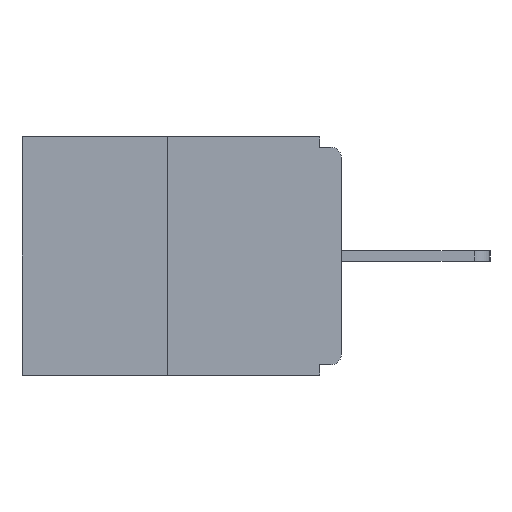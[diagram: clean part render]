
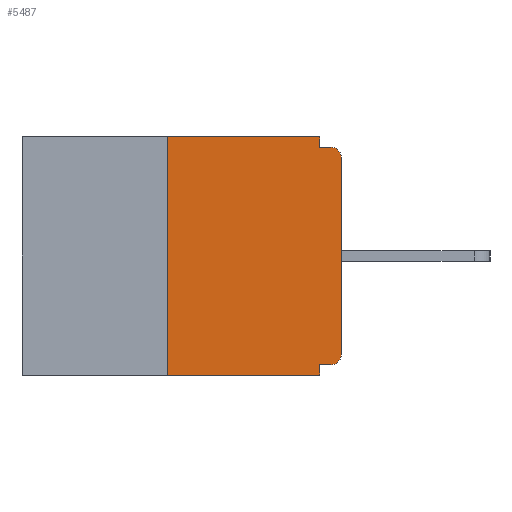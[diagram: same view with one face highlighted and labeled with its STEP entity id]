
A CAD part, left-side view. The second image highlights one B-rep face of the part: STEP entity #5487.
In plain terms, the highlighted planar face has unit normal (-1, 0, 0).
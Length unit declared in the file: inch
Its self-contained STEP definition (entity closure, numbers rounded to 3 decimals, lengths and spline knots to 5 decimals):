
#47 = CARTESIAN_POINT ( 'NONE',  ( 0., 0.015, -0.328 ) ) ;
#153 = CARTESIAN_POINT ( 'NONE',  ( 0., 0., -0.328 ) ) ;
#183 = CARTESIAN_POINT ( 'NONE',  ( 0., 0.46, 0. ) ) ;
#528 = EDGE_CURVE ( 'NONE', #22806, #22956, #4573, .T. ) ;
#566 = CARTESIAN_POINT ( 'NONE',  ( 0., 0., -0.015 ) ) ;
#875 = CARTESIAN_POINT ( 'NONE',  ( 0., 0.031, -0.015 ) ) ;
#1063 = ORIENTED_EDGE ( 'NONE', *, *, #13014, .T. ) ;
#1598 = CIRCLE ( 'NONE', #15785, 0.015 ) ;
#1713 = LINE ( 'NONE', #566, #11301 ) ;
#2596 = ORIENTED_EDGE ( 'NONE', *, *, #18009, .F. ) ;
#2713 = VERTEX_POINT ( 'NONE', #8133 ) ;
#3279 = CARTESIAN_POINT ( 'NONE',  ( 0., 0.031, 0. ) ) ;
#3732 = PLANE ( 'NONE',  #17270 ) ;
#3936 = EDGE_CURVE ( 'NONE', #22615, #22133, #1598, .T. ) ;
#4573 = LINE ( 'NONE', #6725, #20364 ) ;
#4739 = CARTESIAN_POINT ( 'NONE',  ( 0., 0., -0.03 ) ) ;
#4906 = DIRECTION ( 'NONE',  ( 0., 0., -1. ) ) ;
#4944 = DIRECTION ( 'NONE',  ( 0., -1., 0. ) ) ;
#5303 = CARTESIAN_POINT ( 'NONE',  ( 0., 0.015, -0.03 ) ) ;
#5355 = DIRECTION ( 'NONE',  ( -1., 0., 0. ) ) ;
#5487 = ADVANCED_FACE ( 'NONE', ( #7927 ), #3732, .F. ) ;
#5621 = LINE ( 'NONE', #18675, #11233 ) ;
#5684 = DIRECTION ( 'NONE',  ( 0., 0., -1. ) ) ;
#5750 = VERTEX_POINT ( 'NONE', #8669 ) ;
#5790 = VECTOR ( 'NONE', #16634, 39.37008 ) ;
#6542 = EDGE_CURVE ( 'NONE', #11334, #2713, #22577, .T. ) ;
#6725 = CARTESIAN_POINT ( 'NONE',  ( 0., 0.46, 0. ) ) ;
#6993 = CARTESIAN_POINT ( 'NONE',  ( 0., 0.46, -0.343 ) ) ;
#7235 = CARTESIAN_POINT ( 'NONE',  ( 0., 0.031, -0.328 ) ) ;
#7927 = FACE_OUTER_BOUND ( 'NONE', #17029, .T. ) ;
#7964 = EDGE_CURVE ( 'NONE', #22956, #19460, #20913, .T. ) ;
#8133 = CARTESIAN_POINT ( 'NONE',  ( 0., 0., -0.313 ) ) ;
#8654 = ORIENTED_EDGE ( 'NONE', *, *, #14300, .F. ) ;
#8669 = CARTESIAN_POINT ( 'NONE',  ( 0., 0.25, -0.343 ) ) ;
#9293 = LINE ( 'NONE', #153, #14340 ) ;
#10067 = VERTEX_POINT ( 'NONE', #15143 ) ;
#10316 = EDGE_CURVE ( 'NONE', #19460, #22133, #1713, .T. ) ;
#10965 = DIRECTION ( 'NONE',  ( 0., 0., -1. ) ) ;
#11146 = DIRECTION ( 'NONE',  ( 0., 0., 1. ) ) ;
#11233 = VECTOR ( 'NONE', #10965, 39.37008 ) ;
#11301 = VECTOR ( 'NONE', #14036, 39.37008 ) ;
#11334 = VERTEX_POINT ( 'NONE', #47 ) ;
#11351 = LINE ( 'NONE', #18862, #15812 ) ;
#11620 = ORIENTED_EDGE ( 'NONE', *, *, #10316, .F. ) ;
#11762 = EDGE_CURVE ( 'NONE', #18488, #10067, #5621, .T. ) ;
#13014 = EDGE_CURVE ( 'NONE', #5750, #10067, #18652, .T. ) ;
#13365 = ORIENTED_EDGE ( 'NONE', *, *, #6542, .T. ) ;
#14036 = DIRECTION ( 'NONE',  ( 0., -1., 0. ) ) ;
#14300 = EDGE_CURVE ( 'NONE', #5750, #22806, #21024, .T. ) ;
#14340 = VECTOR ( 'NONE', #19371, 39.37008 ) ;
#15002 = DIRECTION ( 'NONE',  ( 0., 0., 1. ) ) ;
#15143 = CARTESIAN_POINT ( 'NONE',  ( 0., 0.031, -0.343 ) ) ;
#15548 = DIRECTION ( 'NONE',  ( 0., 0., -1. ) ) ;
#15574 = DIRECTION ( 'NONE',  ( -1., 0., 0. ) ) ;
#15600 = CARTESIAN_POINT ( 'NONE',  ( 0., 0.015, -0.313 ) ) ;
#15785 = AXIS2_PLACEMENT_3D ( 'NONE', #5303, #5355, #5684 ) ;
#15812 = VECTOR ( 'NONE', #15002, 39.37008 ) ;
#16568 = VECTOR ( 'NONE', #11146, 39.37008 ) ;
#16634 = DIRECTION ( 'NONE',  ( 0., 0., -1. ) ) ;
#17029 = EDGE_LOOP ( 'NONE', ( #18161, #8654, #1063, #17575, #2596, #13365, #24479, #18791, #11620, #20601 ) ) ;
#17217 = CARTESIAN_POINT ( 'NONE',  ( 0., 0.031, 0. ) ) ;
#17270 = AXIS2_PLACEMENT_3D ( 'NONE', #183, #23606, #4906 ) ;
#17575 = ORIENTED_EDGE ( 'NONE', *, *, #11762, .F. ) ;
#18009 = EDGE_CURVE ( 'NONE', #11334, #18488, #9293, .T. ) ;
#18161 = ORIENTED_EDGE ( 'NONE', *, *, #528, .F. ) ;
#18488 = VERTEX_POINT ( 'NONE', #7235 ) ;
#18652 = LINE ( 'NONE', #6993, #22352 ) ;
#18654 = CARTESIAN_POINT ( 'NONE',  ( 0., 0.25, 0. ) ) ;
#18675 = CARTESIAN_POINT ( 'NONE',  ( 0., 0.031, -0.343 ) ) ;
#18791 = ORIENTED_EDGE ( 'NONE', *, *, #3936, .T. ) ;
#18862 = CARTESIAN_POINT ( 'NONE',  ( 0., 0., 0. ) ) ;
#19371 = DIRECTION ( 'NONE',  ( 0., 1., 0. ) ) ;
#19460 = VERTEX_POINT ( 'NONE', #875 ) ;
#20364 = VECTOR ( 'NONE', #4944, 39.37008 ) ;
#20601 = ORIENTED_EDGE ( 'NONE', *, *, #7964, .F. ) ;
#20651 = CARTESIAN_POINT ( 'NONE',  ( 0., 0.25, 0. ) ) ;
#20913 = LINE ( 'NONE', #3279, #5790 ) ;
#21024 = LINE ( 'NONE', #20651, #16568 ) ;
#22083 = DIRECTION ( 'NONE',  ( 0., -1., 0. ) ) ;
#22133 = VERTEX_POINT ( 'NONE', #23952 ) ;
#22352 = VECTOR ( 'NONE', #22083, 39.37008 ) ;
#22577 = CIRCLE ( 'NONE', #24539, 0.015 ) ;
#22615 = VERTEX_POINT ( 'NONE', #4739 ) ;
#22806 = VERTEX_POINT ( 'NONE', #18654 ) ;
#22956 = VERTEX_POINT ( 'NONE', #17217 ) ;
#23606 = DIRECTION ( 'NONE',  ( 1., 0., 0. ) ) ;
#23952 = CARTESIAN_POINT ( 'NONE',  ( 0., 0.015, -0.015 ) ) ;
#24163 = EDGE_CURVE ( 'NONE', #2713, #22615, #11351, .T. ) ;
#24479 = ORIENTED_EDGE ( 'NONE', *, *, #24163, .T. ) ;
#24539 = AXIS2_PLACEMENT_3D ( 'NONE', #15600, #15574, #15548 ) ;
